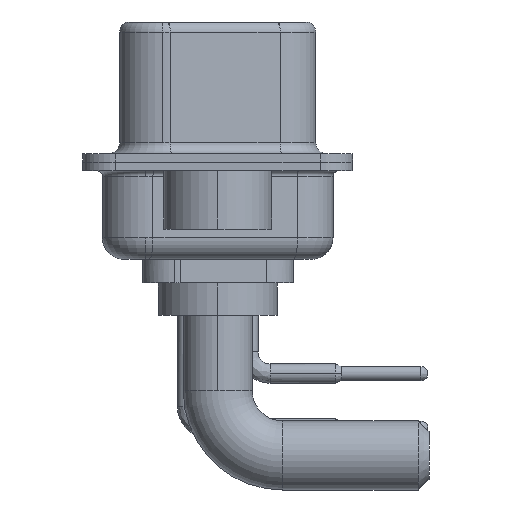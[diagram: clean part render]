
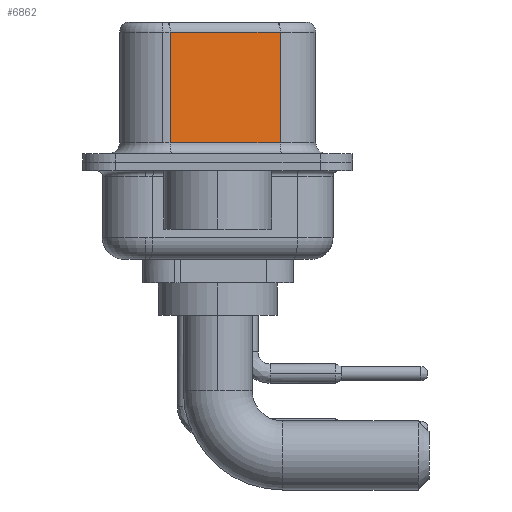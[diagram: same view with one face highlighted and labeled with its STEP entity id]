
A CAD part, left-side view. The second image highlights one B-rep face of the part: STEP entity #6862.
In plain terms, the highlighted planar face has unit normal (-0.985, -0.174, 0).
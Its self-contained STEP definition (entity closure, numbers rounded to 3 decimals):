
#494 = DIRECTION ( 'NONE',  ( -0.174, 0.985, 0. ) ) ;
#565 = VECTOR ( 'NONE', #1446, 1000. ) ;
#586 = EDGE_CURVE ( 'NONE', #27348, #16325, #8373, .T. ) ;
#1446 = DIRECTION ( 'NONE',  ( 0., 0., -1. ) ) ;
#1706 = ORIENTED_EDGE ( 'NONE', *, *, #586, .F. ) ;
#1908 = VERTEX_POINT ( 'NONE', #15220 ) ;
#3051 = EDGE_CURVE ( 'NONE', #10943, #1908, #3597, .T. ) ;
#3597 = LINE ( 'NONE', #12232, #23505 ) ;
#4008 = LINE ( 'NONE', #21246, #13754 ) ;
#5400 = ORIENTED_EDGE ( 'NONE', *, *, #20214, .T. ) ;
#5802 = EDGE_LOOP ( 'NONE', ( #1706, #5400, #24015, #21626 ) ) ;
#6862 = ADVANCED_FACE ( 'NONE', ( #15770 ), #13645, .F. ) ;
#7214 = CARTESIAN_POINT ( 'NONE',  ( 4.58, -2.897, 0.9 ) ) ;
#7406 = CARTESIAN_POINT ( 'NONE',  ( 4.58, -2.897, 6.02 ) ) ;
#7454 = CARTESIAN_POINT ( 'NONE',  ( 4.58, -2.897, 6.02 ) ) ;
#8373 = LINE ( 'NONE', #23228, #565 ) ;
#10943 = VERTEX_POINT ( 'NONE', #19045 ) ;
#12232 = CARTESIAN_POINT ( 'NONE',  ( 3.68, 2.203, 6.52 ) ) ;
#12949 = AXIS2_PLACEMENT_3D ( 'NONE', #20282, #24534, #494 ) ;
#13645 = PLANE ( 'NONE',  #12949 ) ;
#13754 = VECTOR ( 'NONE', #26547, 1000. ) ;
#13864 = VECTOR ( 'NONE', #24700, 1000. ) ;
#15220 = CARTESIAN_POINT ( 'NONE',  ( 3.68, 2.203, 0.9 ) ) ;
#15770 = FACE_OUTER_BOUND ( 'NONE', #5802, .T. ) ;
#16325 = VERTEX_POINT ( 'NONE', #7214 ) ;
#19045 = CARTESIAN_POINT ( 'NONE',  ( 3.68, 2.203, 6.02 ) ) ;
#20214 = EDGE_CURVE ( 'NONE', #27348, #10943, #26813, .T. ) ;
#20282 = CARTESIAN_POINT ( 'NONE',  ( 4.58, -2.897, 6.52 ) ) ;
#21246 = CARTESIAN_POINT ( 'NONE',  ( 4.58, -2.897, 0.9 ) ) ;
#21626 = ORIENTED_EDGE ( 'NONE', *, *, #23825, .T. ) ;
#23228 = CARTESIAN_POINT ( 'NONE',  ( 4.58, -2.897, 6.52 ) ) ;
#23505 = VECTOR ( 'NONE', #25084, 1000. ) ;
#23825 = EDGE_CURVE ( 'NONE', #1908, #16325, #4008, .T. ) ;
#24015 = ORIENTED_EDGE ( 'NONE', *, *, #3051, .T. ) ;
#24534 = DIRECTION ( 'NONE',  ( 0.985, 0.174, 0. ) ) ;
#24700 = DIRECTION ( 'NONE',  ( -0.174, 0.985, 0. ) ) ;
#25084 = DIRECTION ( 'NONE',  ( 0., 0., -1. ) ) ;
#26547 = DIRECTION ( 'NONE',  ( 0.174, -0.985, 0. ) ) ;
#26813 = LINE ( 'NONE', #7454, #13864 ) ;
#27348 = VERTEX_POINT ( 'NONE', #7406 ) ;
